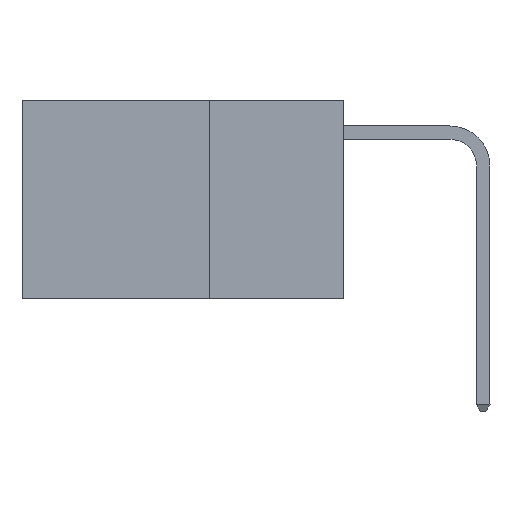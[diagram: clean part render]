
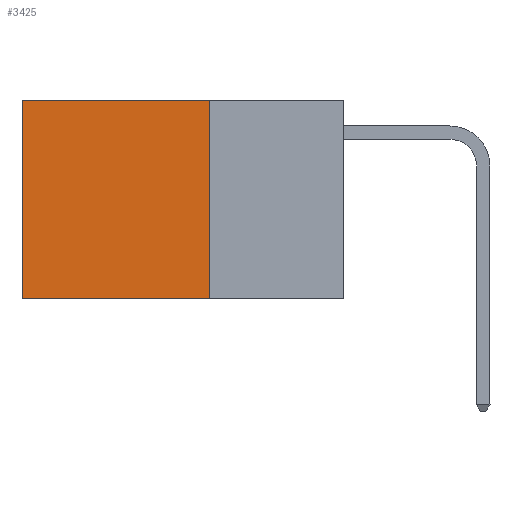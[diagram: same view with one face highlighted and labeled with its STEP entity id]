
A CAD part, left-side view. The second image highlights one B-rep face of the part: STEP entity #3425.
In plain terms, the highlighted planar face has unit normal (-1, 0, 0).
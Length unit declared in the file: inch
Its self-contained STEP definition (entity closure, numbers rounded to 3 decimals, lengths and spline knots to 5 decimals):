
#346 = CARTESIAN_POINT ( 'NONE',  ( 0.2625, 0.25, 0. ) ) ;
#1158 = DIRECTION ( 'NONE',  ( 0., 0., -1. ) ) ;
#1470 = ORIENTED_EDGE ( 'NONE', *, *, #3290, .T. ) ;
#1520 = DIRECTION ( 'NONE',  ( 0., 0., -1. ) ) ;
#2247 = ORIENTED_EDGE ( 'NONE', *, *, #7391, .F. ) ;
#2268 = DIRECTION ( 'NONE',  ( 1., 0., 0. ) ) ;
#2645 = VERTEX_POINT ( 'NONE', #346 ) ;
#2701 = VECTOR ( 'NONE', #6868, 39.37008 ) ;
#2824 = LINE ( 'NONE', #5875, #5861 ) ;
#3271 = CARTESIAN_POINT ( 'NONE',  ( 0.2625, 0.6, 0. ) ) ;
#3290 = EDGE_CURVE ( 'NONE', #2645, #6950, #3420, .T. ) ;
#3371 = EDGE_LOOP ( 'NONE', ( #6508, #8809, #2247, #1470 ) ) ;
#3420 = LINE ( 'NONE', #7127, #6440 ) ;
#3425 = ADVANCED_FACE ( 'NONE', ( #9120 ), #9211, .F. ) ;
#3754 = VECTOR ( 'NONE', #1158, 39.37008 ) ;
#4472 = EDGE_CURVE ( 'NONE', #6950, #7800, #9484, .T. ) ;
#4833 = LINE ( 'NONE', #5349, #2701 ) ;
#4856 = VERTEX_POINT ( 'NONE', #7909 ) ;
#4882 = DIRECTION ( 'NONE',  ( 0., 1., 0. ) ) ;
#5349 = CARTESIAN_POINT ( 'NONE',  ( 0.2625, 0.25, -0.37 ) ) ;
#5400 = CARTESIAN_POINT ( 'NONE',  ( 0.2625, 0.25, 0. ) ) ;
#5682 = CARTESIAN_POINT ( 'NONE',  ( 0.2625, 0.6, 0. ) ) ;
#5861 = VECTOR ( 'NONE', #8909, 39.37008 ) ;
#5875 = CARTESIAN_POINT ( 'NONE',  ( 0.2625, 0.25, 0. ) ) ;
#6440 = VECTOR ( 'NONE', #4882, 39.37008 ) ;
#6508 = ORIENTED_EDGE ( 'NONE', *, *, #4472, .T. ) ;
#6868 = DIRECTION ( 'NONE',  ( 0., 1., 0. ) ) ;
#6950 = VERTEX_POINT ( 'NONE', #3271 ) ;
#7127 = CARTESIAN_POINT ( 'NONE',  ( 0.2625, 0.25, 0. ) ) ;
#7232 = AXIS2_PLACEMENT_3D ( 'NONE', #5400, #2268, #1520 ) ;
#7391 = EDGE_CURVE ( 'NONE', #2645, #4856, #2824, .T. ) ;
#7661 = CARTESIAN_POINT ( 'NONE',  ( 0.2625, 0.6, -0.37 ) ) ;
#7800 = VERTEX_POINT ( 'NONE', #7661 ) ;
#7909 = CARTESIAN_POINT ( 'NONE',  ( 0.2625, 0.25, -0.37 ) ) ;
#8809 = ORIENTED_EDGE ( 'NONE', *, *, #9726, .F. ) ;
#8909 = DIRECTION ( 'NONE',  ( 0., 0., -1. ) ) ;
#9120 = FACE_OUTER_BOUND ( 'NONE', #3371, .T. ) ;
#9211 = PLANE ( 'NONE',  #7232 ) ;
#9484 = LINE ( 'NONE', #5682, #3754 ) ;
#9726 = EDGE_CURVE ( 'NONE', #4856, #7800, #4833, .T. ) ;
